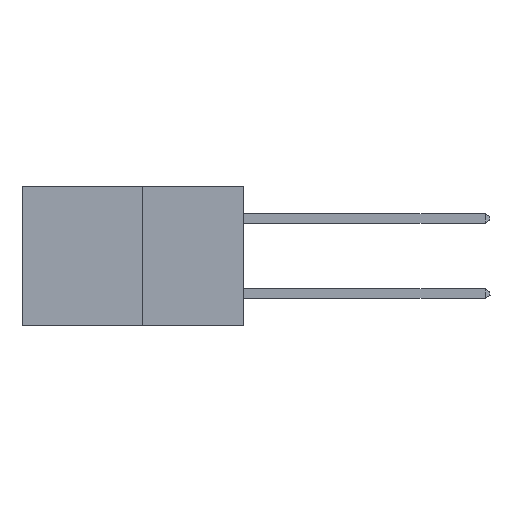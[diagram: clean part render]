
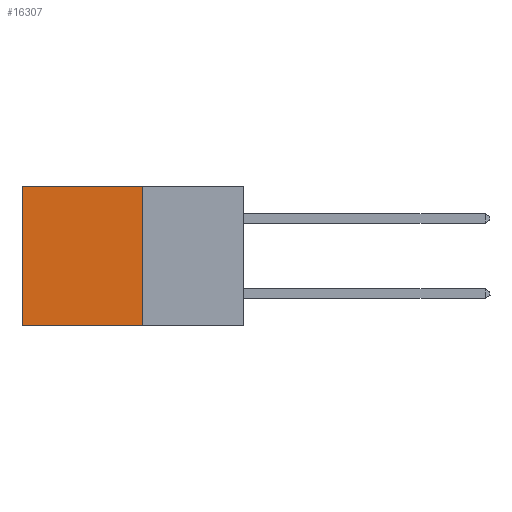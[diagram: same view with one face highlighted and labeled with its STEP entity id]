
A CAD part, left-side view. The second image highlights one B-rep face of the part: STEP entity #16307.
In plain terms, the highlighted planar face has unit normal (-1, 0, 0).
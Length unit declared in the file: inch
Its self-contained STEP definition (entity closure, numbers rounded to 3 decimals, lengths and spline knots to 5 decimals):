
#301 = CARTESIAN_POINT ( 'NONE',  ( 0.277, 0.27, 0. ) ) ;
#390 = DIRECTION ( 'NONE',  ( 0., 1., 0. ) ) ;
#642 = VERTEX_POINT ( 'NONE', #4556 ) ;
#1213 = EDGE_CURVE ( 'NONE', #18026, #7937, #5820, .T. ) ;
#1557 = VERTEX_POINT ( 'NONE', #4698 ) ;
#1679 = ORIENTED_EDGE ( 'NONE', *, *, #20644, .F. ) ;
#1754 = DIRECTION ( 'NONE',  ( 0., 1., 0. ) ) ;
#1837 = EDGE_CURVE ( 'NONE', #642, #18026, #11831, .T. ) ;
#1930 = VECTOR ( 'NONE', #390, 39.37008 ) ;
#3401 = ORIENTED_EDGE ( 'NONE', *, *, #12549, .F. ) ;
#4556 = CARTESIAN_POINT ( 'NONE',  ( 0.277, 0.27, 0. ) ) ;
#4698 = CARTESIAN_POINT ( 'NONE',  ( 0.277, 0.27, -0.37 ) ) ;
#5820 = LINE ( 'NONE', #10901, #18707 ) ;
#6730 = DIRECTION ( 'NONE',  ( 0., 0., -1. ) ) ;
#7213 = DIRECTION ( 'NONE',  ( 0., 0., -1. ) ) ;
#7758 = FACE_OUTER_BOUND ( 'NONE', #16659, .T. ) ;
#7937 = VERTEX_POINT ( 'NONE', #9493 ) ;
#9066 = LINE ( 'NONE', #20858, #22254 ) ;
#9493 = CARTESIAN_POINT ( 'NONE',  ( 0.277, 0.59, -0.37 ) ) ;
#9559 = ORIENTED_EDGE ( 'NONE', *, *, #1213, .T. ) ;
#10688 = PLANE ( 'NONE',  #11063 ) ;
#10901 = CARTESIAN_POINT ( 'NONE',  ( 0.277, 0.59, -0.37 ) ) ;
#11063 = AXIS2_PLACEMENT_3D ( 'NONE', #14221, #17765, #7213 ) ;
#11831 = LINE ( 'NONE', #301, #1930 ) ;
#11978 = VECTOR ( 'NONE', #6730, 39.37008 ) ;
#12549 = EDGE_CURVE ( 'NONE', #1557, #7937, #9066, .T. ) ;
#13718 = CARTESIAN_POINT ( 'NONE',  ( 0.277, 0.27, -0.37 ) ) ;
#14221 = CARTESIAN_POINT ( 'NONE',  ( 0.277, 0.27, -0.37 ) ) ;
#14323 = ORIENTED_EDGE ( 'NONE', *, *, #1837, .T. ) ;
#16307 = ADVANCED_FACE ( 'NONE', ( #7758 ), #10688, .F. ) ;
#16659 = EDGE_LOOP ( 'NONE', ( #9559, #3401, #1679, #14323 ) ) ;
#16686 = LINE ( 'NONE', #13718, #11978 ) ;
#17705 = DIRECTION ( 'NONE',  ( 0., 0., -1. ) ) ;
#17765 = DIRECTION ( 'NONE',  ( 1., 0., 0. ) ) ;
#18026 = VERTEX_POINT ( 'NONE', #22046 ) ;
#18707 = VECTOR ( 'NONE', #17705, 39.37008 ) ;
#20644 = EDGE_CURVE ( 'NONE', #642, #1557, #16686, .T. ) ;
#20858 = CARTESIAN_POINT ( 'NONE',  ( 0.277, 0.27, -0.37 ) ) ;
#22046 = CARTESIAN_POINT ( 'NONE',  ( 0.277, 0.59, 0. ) ) ;
#22254 = VECTOR ( 'NONE', #1754, 39.37008 ) ;
